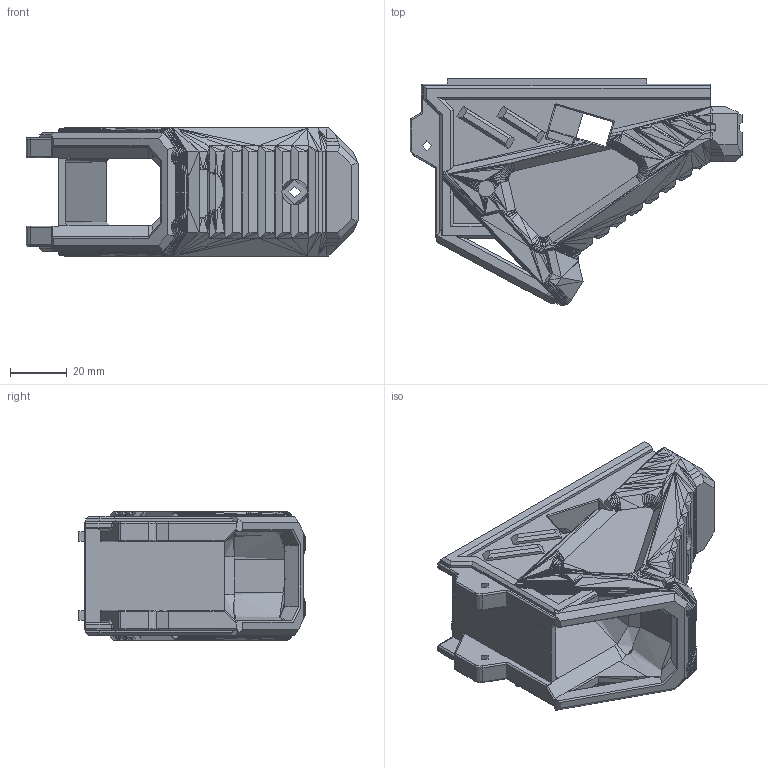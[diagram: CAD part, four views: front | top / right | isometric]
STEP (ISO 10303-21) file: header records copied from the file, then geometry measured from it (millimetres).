
FILE_DESCRIPTION(/* description */ ('STEP AP214'),/* implementation_level */ '2;1');
FILE_NAME(/* author */ (''),/* organization */ (''),/* preprocessor_version */ 'ST-DEVELOPER v18.1',/* originating_system */ ' ',/* authorisation */ ' ');
FILE_SCHEMA (('AUTOMOTIVE_DESIGN {1 0 10303 214 3 1 1}'));
Length unit declared in the file: metre
Products named in the file (1): bloc2
Bounding box: 116.51 x 79.5 x 44.94 mm (x, y, z)
Volume: 150253.6 mm3
Topology: 1 solids, 2 shells, 1830 faces, 3945 edges, 2124 vertices
Faces by surface type: plane 1673, cylinder 95, bspline 39, torus 17, sphere 6
Full cylindrical faces by diameter (mm): 1.5 x1, 3.4 x2, 4 x2, 9 x1
Entity records: 48330 total; most frequent: CARTESIAN_POINT 10028, ORIENTED_EDGE 7870, DIRECTION 7550, EDGE_CURVE 3935, LINE 3396, VECTOR 3396, VERTEX_POINT 2123, AXIS2_PLACEMENT_3D 2077
